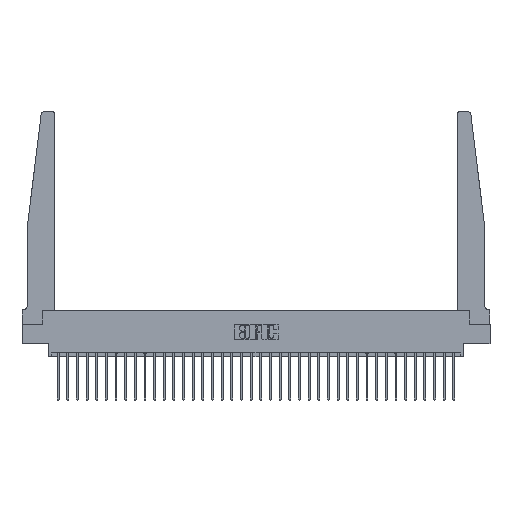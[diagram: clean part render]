
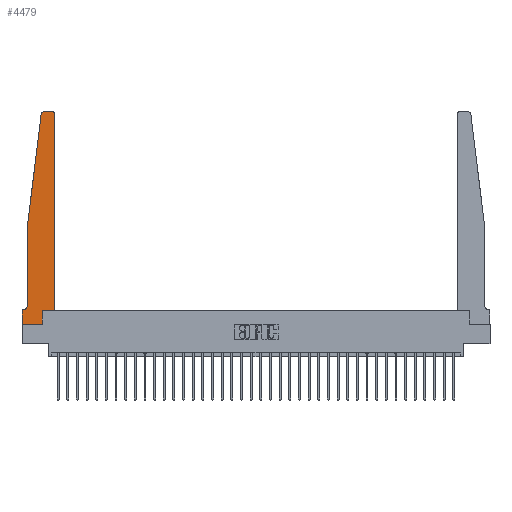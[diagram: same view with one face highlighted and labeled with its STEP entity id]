
A CAD part, top view. The second image highlights one B-rep face of the part: STEP entity #4479.
In plain terms, the highlighted planar face has unit normal (0, 0, 1).
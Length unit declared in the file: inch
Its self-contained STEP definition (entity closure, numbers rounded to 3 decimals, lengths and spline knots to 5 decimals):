
#451 = VERTEX_POINT ( 'NONE', #2057 ) ;
#672 = DIRECTION ( 'NONE',  ( 0., 0., -1. ) ) ;
#756 = DIRECTION ( 'NONE',  ( 1., 0., 0. ) ) ;
#1210 = LINE ( 'NONE', #25084, #8964 ) ;
#1281 = VERTEX_POINT ( 'NONE', #22689 ) ;
#1460 = AXIS2_PLACEMENT_3D ( 'NONE', #5326, #22898, #5655 ) ;
#2057 = CARTESIAN_POINT ( 'NONE',  ( 0.395, 2.75, 0.37 ) ) ;
#2105 = ORIENTED_EDGE ( 'NONE', *, *, #19250, .T. ) ;
#2108 = CARTESIAN_POINT ( 'NONE',  ( 0.24675, 2.72367, 0.37 ) ) ;
#2109 = VERTEX_POINT ( 'NONE', #32753 ) ;
#2473 = LINE ( 'NONE', #30015, #15843 ) ;
#2859 = CARTESIAN_POINT ( 'NONE',  ( 0., 0., 0.37 ) ) ;
#2950 = VECTOR ( 'NONE', #26518, 39.37008 ) ;
#3407 = CARTESIAN_POINT ( 'NONE',  ( 0.27653, 2.75, 0.37 ) ) ;
#3646 = CARTESIAN_POINT ( 'NONE',  ( 0.065, 1.25, 0.37 ) ) ;
#3834 = ORIENTED_EDGE ( 'NONE', *, *, #4764, .T. ) ;
#3947 = CARTESIAN_POINT ( 'NONE',  ( 0.25, 2.75, 0.37 ) ) ;
#4479 = ADVANCED_FACE ( 'NONE', ( #31121 ), #26302, .T. ) ;
#4701 = CARTESIAN_POINT ( 'NONE',  ( 0., 0., 0.37 ) ) ;
#4764 = EDGE_CURVE ( 'NONE', #9846, #22419, #28123, .T. ) ;
#5036 = DIRECTION ( 'NONE',  ( -0.122, -0.992, 0. ) ) ;
#5326 = CARTESIAN_POINT ( 'NONE',  ( 0.395, 2.72, 0.37 ) ) ;
#5402 = EDGE_CURVE ( 'NONE', #451, #24563, #18088, .T. ) ;
#5514 = CARTESIAN_POINT ( 'NONE',  ( 0., 0., 0.37 ) ) ;
#5655 = DIRECTION ( 'NONE',  ( 1., 0., 0. ) ) ;
#5840 = LINE ( 'NONE', #5514, #9477 ) ;
#6005 = ORIENTED_EDGE ( 'NONE', *, *, #23343, .T. ) ;
#6388 = CARTESIAN_POINT ( 'NONE',  ( 0.065, 0.1875, 0.37 ) ) ;
#6679 = DIRECTION ( 'NONE',  ( 0., 0., 1. ) ) ;
#6789 = DIRECTION ( 'NONE',  ( 1., 0., 0. ) ) ;
#6867 = CARTESIAN_POINT ( 'NONE',  ( 0.015, 0.1875, 0.37 ) ) ;
#7333 = ORIENTED_EDGE ( 'NONE', *, *, #17244, .T. ) ;
#8092 = LINE ( 'NONE', #13062, #10654 ) ;
#8253 = DIRECTION ( 'NONE',  ( 0., 1., 0. ) ) ;
#8332 = VERTEX_POINT ( 'NONE', #6867 ) ;
#8348 = CIRCLE ( 'NONE', #1460, 0.03 ) ;
#8964 = VECTOR ( 'NONE', #19590, 39.37008 ) ;
#9317 = VECTOR ( 'NONE', #17483, 39.37008 ) ;
#9477 = VECTOR ( 'NONE', #28581, 39.37008 ) ;
#9616 = CARTESIAN_POINT ( 'NONE',  ( 0.2605, 0., 0.37 ) ) ;
#9846 = VERTEX_POINT ( 'NONE', #2108 ) ;
#10014 = DIRECTION ( 'NONE',  ( 1., 0., 0. ) ) ;
#10654 = VECTOR ( 'NONE', #8253, 39.37008 ) ;
#10725 = DIRECTION ( 'NONE',  ( 0., 0., 1. ) ) ;
#11498 = EDGE_CURVE ( 'NONE', #18028, #1281, #12670, .T. ) ;
#11916 = EDGE_CURVE ( 'NONE', #24563, #9846, #31585, .T. ) ;
#12670 = LINE ( 'NONE', #15327, #9317 ) ;
#12823 = ORIENTED_EDGE ( 'NONE', *, *, #14832, .T. ) ;
#13062 = CARTESIAN_POINT ( 'NONE',  ( 0.2605, 0.18, 0.37 ) ) ;
#13711 = CIRCLE ( 'NONE', #32274, 0.05 ) ;
#14471 = CARTESIAN_POINT ( 'NONE',  ( 0.27653, 2.72, 0.37 ) ) ;
#14832 = EDGE_CURVE ( 'NONE', #28659, #30726, #17297, .T. ) ;
#15137 = ORIENTED_EDGE ( 'NONE', *, *, #29167, .T. ) ;
#15327 = CARTESIAN_POINT ( 'NONE',  ( 0.425, 0.18, 0.37 ) ) ;
#15346 = EDGE_CURVE ( 'NONE', #16832, #8332, #13711, .T. ) ;
#15634 = EDGE_CURVE ( 'NONE', #23661, #18028, #2473, .T. ) ;
#15843 = VECTOR ( 'NONE', #6789, 39.37008 ) ;
#16813 = AXIS2_PLACEMENT_3D ( 'NONE', #31294, #10725, #756 ) ;
#16832 = VERTEX_POINT ( 'NONE', #21111 ) ;
#17244 = EDGE_CURVE ( 'NONE', #2109, #28659, #5840, .T. ) ;
#17297 = LINE ( 'NONE', #4701, #18984 ) ;
#17483 = DIRECTION ( 'NONE',  ( 0., 1., 0. ) ) ;
#18028 = VERTEX_POINT ( 'NONE', #19686 ) ;
#18088 = LINE ( 'NONE', #3947, #2950 ) ;
#18984 = VECTOR ( 'NONE', #10014, 39.37008 ) ;
#19250 = EDGE_CURVE ( 'NONE', #30726, #23661, #8092, .T. ) ;
#19252 = ORIENTED_EDGE ( 'NONE', *, *, #31466, .T. ) ;
#19590 = DIRECTION ( 'NONE',  ( 0., -1., 0. ) ) ;
#19686 = CARTESIAN_POINT ( 'NONE',  ( 0.425, 0.18, 0.37 ) ) ;
#20570 = ORIENTED_EDGE ( 'NONE', *, *, #11916, .T. ) ;
#21111 = CARTESIAN_POINT ( 'NONE',  ( 0.065, 0.2375, 0.37 ) ) ;
#21954 = DIRECTION ( 'NONE',  ( -1., 0., 0. ) ) ;
#22419 = VERTEX_POINT ( 'NONE', #3646 ) ;
#22689 = CARTESIAN_POINT ( 'NONE',  ( 0.425, 2.72, 0.37 ) ) ;
#22898 = DIRECTION ( 'NONE',  ( 0., 0., 1. ) ) ;
#23091 = EDGE_LOOP ( 'NONE', ( #30094, #20570, #3834, #19252, #29002, #6005, #7333, #12823, #2105, #32368, #30502, #15137 ) ) ;
#23343 = EDGE_CURVE ( 'NONE', #8332, #2109, #28961, .T. ) ;
#23445 = CARTESIAN_POINT ( 'NONE',  ( 0.2605, 0.18, 0.37 ) ) ;
#23560 = CARTESIAN_POINT ( 'NONE',  ( 0.015, 0.2375, 0.37 ) ) ;
#23661 = VERTEX_POINT ( 'NONE', #23445 ) ;
#24563 = VERTEX_POINT ( 'NONE', #3407 ) ;
#25084 = CARTESIAN_POINT ( 'NONE',  ( 0.065, 1.25, 0.37 ) ) ;
#25459 = CARTESIAN_POINT ( 'NONE',  ( 0.065, 1.25, 0.37 ) ) ;
#26302 = PLANE ( 'NONE',  #16813 ) ;
#26518 = DIRECTION ( 'NONE',  ( -1., 0., 0. ) ) ;
#27893 = DIRECTION ( 'NONE',  ( -1., 0., 0. ) ) ;
#28123 = LINE ( 'NONE', #25459, #28692 ) ;
#28581 = DIRECTION ( 'NONE',  ( 0., -1., 0. ) ) ;
#28659 = VERTEX_POINT ( 'NONE', #2859 ) ;
#28692 = VECTOR ( 'NONE', #5036, 39.37008 ) ;
#28961 = LINE ( 'NONE', #6388, #32557 ) ;
#29002 = ORIENTED_EDGE ( 'NONE', *, *, #15346, .T. ) ;
#29095 = DIRECTION ( 'NONE',  ( 1., 0., 0. ) ) ;
#29167 = EDGE_CURVE ( 'NONE', #1281, #451, #8348, .T. ) ;
#30015 = CARTESIAN_POINT ( 'NONE',  ( 0.425, 0.18, 0.37 ) ) ;
#30094 = ORIENTED_EDGE ( 'NONE', *, *, #5402, .T. ) ;
#30502 = ORIENTED_EDGE ( 'NONE', *, *, #11498, .T. ) ;
#30726 = VERTEX_POINT ( 'NONE', #9616 ) ;
#31121 = FACE_OUTER_BOUND ( 'NONE', #23091, .T. ) ;
#31294 = CARTESIAN_POINT ( 'NONE',  ( 0., 0.1875, 0.37 ) ) ;
#31466 = EDGE_CURVE ( 'NONE', #22419, #16832, #1210, .T. ) ;
#31585 = CIRCLE ( 'NONE', #32646, 0.03 ) ;
#32274 = AXIS2_PLACEMENT_3D ( 'NONE', #23560, #672, #27893 ) ;
#32368 = ORIENTED_EDGE ( 'NONE', *, *, #15634, .T. ) ;
#32557 = VECTOR ( 'NONE', #21954, 39.37008 ) ;
#32646 = AXIS2_PLACEMENT_3D ( 'NONE', #14471, #6679, #29095 ) ;
#32753 = CARTESIAN_POINT ( 'NONE',  ( 0., 0.1875, 0.37 ) ) ;
